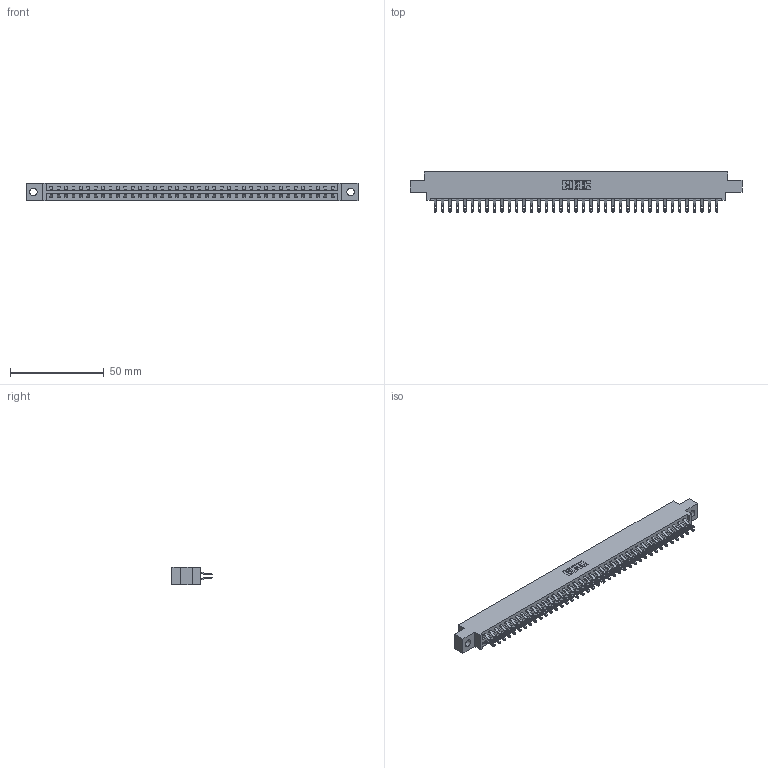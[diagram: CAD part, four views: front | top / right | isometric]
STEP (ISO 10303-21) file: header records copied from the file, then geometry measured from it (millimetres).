
FILE_DESCRIPTION (( 'STEP AP203' ), '1' );
FILE_NAME ('387-078-555-804.STEP', '2018-09-23T17:28:06', ( '' ), ( '' ), 'SwSTEP 2.0', 'SolidWorks 2016', '' );
FILE_SCHEMA (( 'CONFIG_CONTROL_DESIGN' ));
Length unit declared in the file: inch
Products named in the file (3): 337 Part_0.170 Offset - 0.156 Dia-TH; 345-292-001_555 Tail; 387-078-555-804
Assembly tree (79 placements, depth 2):
  387-078-555-804
    337 Part_0.170 Offset - 0.156 Dia-TH
    345-292-001_555 Tail  x78
Bounding box: 177.55 x 21.47 x 9.4 mm (x, y, z)
Volume: 18692.2 mm3; surface area: 21860.2 mm2
Topology: 79 solids, 79 shells, 4798 faces, 15065 edges, 10042 vertices
Faces by surface type: plane 2882, cylinder 1916
Entity records: 31087 total; most frequent: CARTESIAN_POINT 5276, ORIENTED_EDGE 5182, DIRECTION 4463, EDGE_CURVE 2591, LINE 2443, VECTOR 2443, VERTEX_POINT 1726, AXIS2_PLACEMENT_3D 1010
